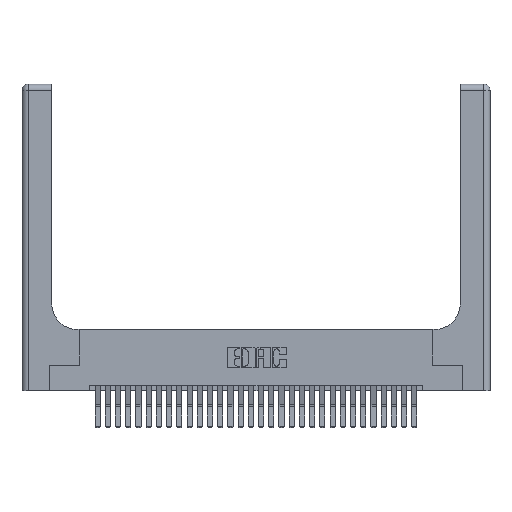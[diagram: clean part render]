
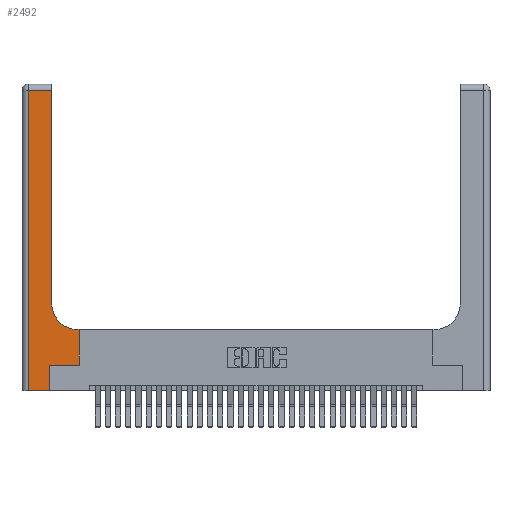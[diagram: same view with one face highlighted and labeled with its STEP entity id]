
A CAD part, top view. The second image highlights one B-rep face of the part: STEP entity #2492.
In plain terms, the highlighted planar face has unit normal (0, 0, 1).
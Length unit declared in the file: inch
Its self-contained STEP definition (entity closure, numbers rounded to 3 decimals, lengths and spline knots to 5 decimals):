
#346 = ORIENTED_EDGE ( 'NONE', *, *, #2434, .T. ) ;
#732 = CARTESIAN_POINT ( 'NONE',  ( 0.06, 0., 0.37 ) ) ;
#2127 = ORIENTED_EDGE ( 'NONE', *, *, #17644, .T. ) ;
#2434 = EDGE_CURVE ( 'NONE', #29906, #18316, #7915, .T. ) ;
#2492 = ADVANCED_FACE ( 'NONE', ( #17900 ), #11798, .F. ) ;
#2522 = VECTOR ( 'NONE', #7693, 39.37008 ) ;
#3140 = LINE ( 'NONE', #15557, #15089 ) ;
#3886 = VERTEX_POINT ( 'NONE', #4989 ) ;
#3967 = DIRECTION ( 'NONE',  ( -1., 0., 0. ) ) ;
#4651 = VECTOR ( 'NONE', #3967, 39.37008 ) ;
#4667 = DIRECTION ( 'NONE',  ( 0., 1., 0. ) ) ;
#4989 = CARTESIAN_POINT ( 'NONE',  ( 0.2915, 0.85, 0.37 ) ) ;
#5027 = EDGE_CURVE ( 'NONE', #23059, #29712, #19252, .T. ) ;
#5233 = VECTOR ( 'NONE', #27873, 39.37008 ) ;
#5307 = AXIS2_PLACEMENT_3D ( 'NONE', #16835, #5897, #22101 ) ;
#5846 = EDGE_CURVE ( 'NONE', #18316, #19847, #16185, .T. ) ;
#5848 = DIRECTION ( 'NONE',  ( 1., 0., 0. ) ) ;
#5897 = DIRECTION ( 'NONE',  ( 0., 0., -1. ) ) ;
#6041 = CARTESIAN_POINT ( 'NONE',  ( 0.5585, 0.6, 0.37 ) ) ;
#7433 = CARTESIAN_POINT ( 'NONE',  ( 0.269, 0.25, 0.37 ) ) ;
#7494 = CARTESIAN_POINT ( 'NONE',  ( 0.2915, 0.6, 0.37 ) ) ;
#7531 = EDGE_CURVE ( 'NONE', #29712, #24150, #28665, .T. ) ;
#7640 = DIRECTION ( 'NONE',  ( 1., 0., 0. ) ) ;
#7693 = DIRECTION ( 'NONE',  ( -1., 0., 0. ) ) ;
#7748 = EDGE_CURVE ( 'NONE', #3886, #23059, #3140, .T. ) ;
#7915 = LINE ( 'NONE', #28784, #18681 ) ;
#9628 = VECTOR ( 'NONE', #7640, 39.37008 ) ;
#10418 = EDGE_CURVE ( 'NONE', #29218, #3886, #30624, .T. ) ;
#10978 = LINE ( 'NONE', #7494, #2522 ) ;
#11798 = PLANE ( 'NONE',  #5307 ) ;
#13764 = ORIENTED_EDGE ( 'NONE', *, *, #23584, .T. ) ;
#14948 = CARTESIAN_POINT ( 'NONE',  ( 0.269, 0.25, 0.37 ) ) ;
#15089 = VECTOR ( 'NONE', #27605, 39.37008 ) ;
#15557 = CARTESIAN_POINT ( 'NONE',  ( 0.2915, 3., 0.37 ) ) ;
#16185 = LINE ( 'NONE', #7433, #9628 ) ;
#16835 = CARTESIAN_POINT ( 'NONE',  ( 0., 3., 0.37 ) ) ;
#17644 = EDGE_CURVE ( 'NONE', #24150, #29906, #19203, .T. ) ;
#17709 = CARTESIAN_POINT ( 'NONE',  ( 0.2915, 2.94, 0.37 ) ) ;
#17877 = CARTESIAN_POINT ( 'NONE',  ( 0.5415, 0.6, 0.37 ) ) ;
#17900 = FACE_OUTER_BOUND ( 'NONE', #20358, .T. ) ;
#17948 = CARTESIAN_POINT ( 'NONE',  ( 0.269, 0., 0.37 ) ) ;
#18316 = VERTEX_POINT ( 'NONE', #14948 ) ;
#18447 = VECTOR ( 'NONE', #23884, 39.37008 ) ;
#18681 = VECTOR ( 'NONE', #4667, 39.37008 ) ;
#18885 = CARTESIAN_POINT ( 'NONE',  ( 0., 2.94, 0.37 ) ) ;
#18983 = LINE ( 'NONE', #28379, #23210 ) ;
#19203 = LINE ( 'NONE', #23990, #18447 ) ;
#19252 = LINE ( 'NONE', #18885, #4651 ) ;
#19847 = VERTEX_POINT ( 'NONE', #27007 ) ;
#20038 = ORIENTED_EDGE ( 'NONE', *, *, #5027, .T. ) ;
#20358 = EDGE_LOOP ( 'NONE', ( #30847, #20038, #23963, #2127, #346, #22426, #20506, #13764, #24253 ) ) ;
#20506 = ORIENTED_EDGE ( 'NONE', *, *, #21055, .T. ) ;
#21055 = EDGE_CURVE ( 'NONE', #19847, #26985, #18983, .T. ) ;
#22101 = DIRECTION ( 'NONE',  ( -1., 0., 0. ) ) ;
#22426 = ORIENTED_EDGE ( 'NONE', *, *, #5846, .T. ) ;
#23001 = AXIS2_PLACEMENT_3D ( 'NONE', #27928, #30274, #5848 ) ;
#23059 = VERTEX_POINT ( 'NONE', #17709 ) ;
#23210 = VECTOR ( 'NONE', #28053, 39.37008 ) ;
#23584 = EDGE_CURVE ( 'NONE', #26985, #29218, #10978, .T. ) ;
#23884 = DIRECTION ( 'NONE',  ( 1., 0., 0. ) ) ;
#23963 = ORIENTED_EDGE ( 'NONE', *, *, #7531, .T. ) ;
#23990 = CARTESIAN_POINT ( 'NONE',  ( 0., 0., 0.37 ) ) ;
#24150 = VERTEX_POINT ( 'NONE', #732 ) ;
#24253 = ORIENTED_EDGE ( 'NONE', *, *, #10418, .T. ) ;
#26501 = CARTESIAN_POINT ( 'NONE',  ( 0.06, 2.94, 0.37 ) ) ;
#26985 = VERTEX_POINT ( 'NONE', #6041 ) ;
#27007 = CARTESIAN_POINT ( 'NONE',  ( 0.5585, 0.25, 0.37 ) ) ;
#27605 = DIRECTION ( 'NONE',  ( 0., 1., 0. ) ) ;
#27660 = CARTESIAN_POINT ( 'NONE',  ( 0.06, 3., 0.37 ) ) ;
#27873 = DIRECTION ( 'NONE',  ( 0., -1., 0. ) ) ;
#27928 = CARTESIAN_POINT ( 'NONE',  ( 0.5415, 0.85, 0.37 ) ) ;
#28053 = DIRECTION ( 'NONE',  ( 0., 1., 0. ) ) ;
#28379 = CARTESIAN_POINT ( 'NONE',  ( 0.5585, 0.25, 0.37 ) ) ;
#28665 = LINE ( 'NONE', #27660, #5233 ) ;
#28784 = CARTESIAN_POINT ( 'NONE',  ( 0.269, 0., 0.37 ) ) ;
#29218 = VERTEX_POINT ( 'NONE', #17877 ) ;
#29712 = VERTEX_POINT ( 'NONE', #26501 ) ;
#29906 = VERTEX_POINT ( 'NONE', #17948 ) ;
#30274 = DIRECTION ( 'NONE',  ( 0., 0., -1. ) ) ;
#30624 = CIRCLE ( 'NONE', #23001, 0.25 ) ;
#30847 = ORIENTED_EDGE ( 'NONE', *, *, #7748, .T. ) ;
